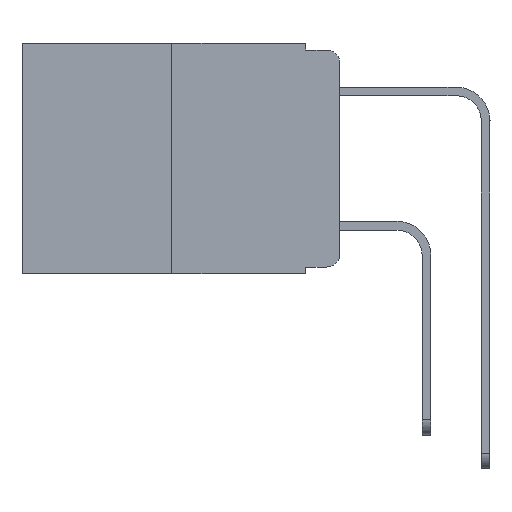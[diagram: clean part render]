
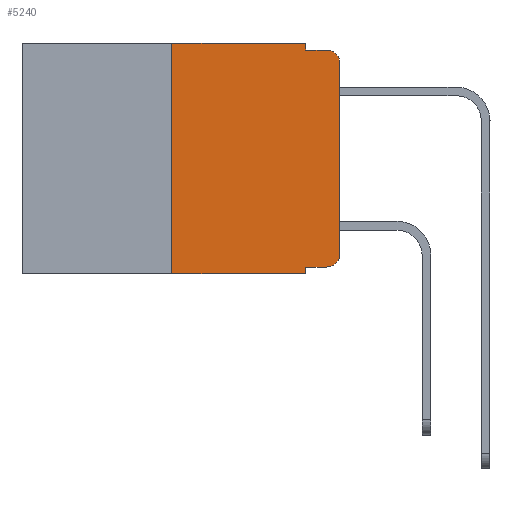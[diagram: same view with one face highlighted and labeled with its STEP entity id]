
A CAD part, left-side view. The second image highlights one B-rep face of the part: STEP entity #5240.
In plain terms, the highlighted planar face has unit normal (-1, 0, 0).
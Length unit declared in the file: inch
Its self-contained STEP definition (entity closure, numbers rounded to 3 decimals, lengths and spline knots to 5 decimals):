
#1533 = ORIENTED_EDGE ( 'NONE', *, *, #8815, .F. ) ;
#1747 = CARTESIAN_POINT ( 'NONE',  ( 0., 0., -0.03 ) ) ;
#1810 = ORIENTED_EDGE ( 'NONE', *, *, #10139, .T. ) ;
#2060 = EDGE_CURVE ( 'NONE', #18328, #8522, #8891, .T. ) ;
#2128 = CARTESIAN_POINT ( 'NONE',  ( 0., 0.051, 0. ) ) ;
#2239 = DIRECTION ( 'NONE',  ( 0., 0., -1. ) ) ;
#2610 = LINE ( 'NONE', #15475, #22815 ) ;
#2698 = CARTESIAN_POINT ( 'NONE',  ( 0., 0., -0.313 ) ) ;
#2752 = VECTOR ( 'NONE', #2862, 39.37008 ) ;
#2862 = DIRECTION ( 'NONE',  ( 0., -1., 0. ) ) ;
#3102 = VERTEX_POINT ( 'NONE', #7751 ) ;
#3451 = EDGE_CURVE ( 'NONE', #23887, #3102, #19785, .T. ) ;
#3572 = VECTOR ( 'NONE', #2239, 39.37008 ) ;
#4348 = CARTESIAN_POINT ( 'NONE',  ( 0., 0.051, 0. ) ) ;
#4382 = DIRECTION ( 'NONE',  ( 0., -1., 0. ) ) ;
#4499 = FACE_OUTER_BOUND ( 'NONE', #17640, .T. ) ;
#4796 = EDGE_CURVE ( 'NONE', #14003, #22821, #2610, .T. ) ;
#5094 = VERTEX_POINT ( 'NONE', #2698 ) ;
#5240 = ADVANCED_FACE ( 'NONE', ( #4499 ), #23392, .F. ) ;
#5457 = CARTESIAN_POINT ( 'NONE',  ( 0., 0.051, -0.343 ) ) ;
#5763 = ORIENTED_EDGE ( 'NONE', *, *, #2060, .F. ) ;
#5827 = CARTESIAN_POINT ( 'NONE',  ( 0., 0., 0. ) ) ;
#5852 = CARTESIAN_POINT ( 'NONE',  ( 0., 0.02, -0.313 ) ) ;
#6568 = LINE ( 'NONE', #16178, #22658 ) ;
#7751 = CARTESIAN_POINT ( 'NONE',  ( 0., 0.25, 0. ) ) ;
#7842 = AXIS2_PLACEMENT_3D ( 'NONE', #9886, #11865, #8711 ) ;
#7849 = DIRECTION ( 'NONE',  ( 0., 0., -1. ) ) ;
#8055 = CARTESIAN_POINT ( 'NONE',  ( 0., 0.02, -0.333 ) ) ;
#8115 = LINE ( 'NONE', #22363, #2752 ) ;
#8431 = CARTESIAN_POINT ( 'NONE',  ( 0., 0.02, -0.03 ) ) ;
#8522 = VERTEX_POINT ( 'NONE', #5457 ) ;
#8711 = DIRECTION ( 'NONE',  ( 0., 0., -1. ) ) ;
#8804 = ORIENTED_EDGE ( 'NONE', *, *, #4796, .F. ) ;
#8815 = EDGE_CURVE ( 'NONE', #22821, #14455, #6568, .T. ) ;
#8891 = LINE ( 'NONE', #4348, #3572 ) ;
#8999 = EDGE_CURVE ( 'NONE', #3102, #14003, #8115, .T. ) ;
#9661 = ORIENTED_EDGE ( 'NONE', *, *, #11441, .T. ) ;
#9886 = CARTESIAN_POINT ( 'NONE',  ( 0., 0.473, 0. ) ) ;
#10139 = EDGE_CURVE ( 'NONE', #22286, #14455, #14165, .T. ) ;
#10408 = DIRECTION ( 'NONE',  ( 0., 0., -1. ) ) ;
#10596 = AXIS2_PLACEMENT_3D ( 'NONE', #5852, #19522, #7849 ) ;
#10731 = DIRECTION ( 'NONE',  ( 0., -1., 0. ) ) ;
#11441 = EDGE_CURVE ( 'NONE', #5094, #22286, #20442, .T. ) ;
#11781 = DIRECTION ( 'NONE',  ( 0., 0., 1. ) ) ;
#11849 = DIRECTION ( 'NONE',  ( 0., -1., 0. ) ) ;
#11865 = DIRECTION ( 'NONE',  ( 1., 0., 0. ) ) ;
#12547 = ORIENTED_EDGE ( 'NONE', *, *, #21317, .T. ) ;
#13021 = CARTESIAN_POINT ( 'NONE',  ( 0., 0.25, -0.343 ) ) ;
#13091 = CARTESIAN_POINT ( 'NONE',  ( 0., 0.02, -0.01 ) ) ;
#13319 = CARTESIAN_POINT ( 'NONE',  ( 0., 0.051, -0.01 ) ) ;
#13333 = VECTOR ( 'NONE', #11849, 39.37008 ) ;
#13672 = CARTESIAN_POINT ( 'NONE',  ( 0., 0.25, 0. ) ) ;
#14003 = VERTEX_POINT ( 'NONE', #2128 ) ;
#14165 = CIRCLE ( 'NONE', #20937, 0.02 ) ;
#14455 = VERTEX_POINT ( 'NONE', #13091 ) ;
#15100 = VECTOR ( 'NONE', #10731, 39.37008 ) ;
#15240 = VECTOR ( 'NONE', #24865, 39.37008 ) ;
#15307 = VECTOR ( 'NONE', #11781, 39.37008 ) ;
#15475 = CARTESIAN_POINT ( 'NONE',  ( 0., 0.051, 0. ) ) ;
#16178 = CARTESIAN_POINT ( 'NONE',  ( 0., 0.051, -0.01 ) ) ;
#16308 = LINE ( 'NONE', #20395, #15100 ) ;
#17086 = ORIENTED_EDGE ( 'NONE', *, *, #22257, .T. ) ;
#17640 = EDGE_LOOP ( 'NONE', ( #9661, #1810, #1533, #8804, #21251, #20969, #12547, #5763, #19225, #17086 ) ) ;
#18094 = CIRCLE ( 'NONE', #10596, 0.02 ) ;
#18328 = VERTEX_POINT ( 'NONE', #20273 ) ;
#19078 = LINE ( 'NONE', #21458, #13333 ) ;
#19225 = ORIENTED_EDGE ( 'NONE', *, *, #23548, .T. ) ;
#19522 = DIRECTION ( 'NONE',  ( -1., 0., 0. ) ) ;
#19785 = LINE ( 'NONE', #13672, #15240 ) ;
#19791 = DIRECTION ( 'NONE',  ( 0., 0., -1. ) ) ;
#20273 = CARTESIAN_POINT ( 'NONE',  ( 0., 0.051, -0.333 ) ) ;
#20395 = CARTESIAN_POINT ( 'NONE',  ( 0., 0.473, -0.343 ) ) ;
#20442 = LINE ( 'NONE', #5827, #15307 ) ;
#20937 = AXIS2_PLACEMENT_3D ( 'NONE', #8431, #21971, #10408 ) ;
#20969 = ORIENTED_EDGE ( 'NONE', *, *, #3451, .F. ) ;
#21251 = ORIENTED_EDGE ( 'NONE', *, *, #8999, .F. ) ;
#21317 = EDGE_CURVE ( 'NONE', #23887, #8522, #16308, .T. ) ;
#21458 = CARTESIAN_POINT ( 'NONE',  ( 0., 0.051, -0.333 ) ) ;
#21971 = DIRECTION ( 'NONE',  ( -1., 0., 0. ) ) ;
#22257 = EDGE_CURVE ( 'NONE', #25386, #5094, #18094, .T. ) ;
#22286 = VERTEX_POINT ( 'NONE', #1747 ) ;
#22363 = CARTESIAN_POINT ( 'NONE',  ( 0., 0.473, 0. ) ) ;
#22658 = VECTOR ( 'NONE', #4382, 39.37008 ) ;
#22815 = VECTOR ( 'NONE', #19791, 39.37008 ) ;
#22821 = VERTEX_POINT ( 'NONE', #13319 ) ;
#23392 = PLANE ( 'NONE',  #7842 ) ;
#23548 = EDGE_CURVE ( 'NONE', #18328, #25386, #19078, .T. ) ;
#23887 = VERTEX_POINT ( 'NONE', #13021 ) ;
#24865 = DIRECTION ( 'NONE',  ( 0., 0., 1. ) ) ;
#25386 = VERTEX_POINT ( 'NONE', #8055 ) ;
